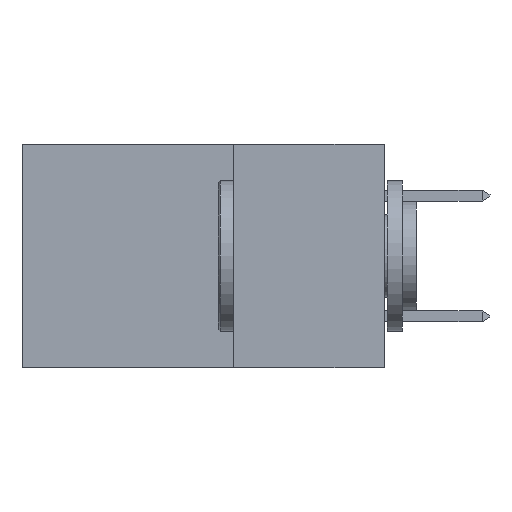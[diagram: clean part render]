
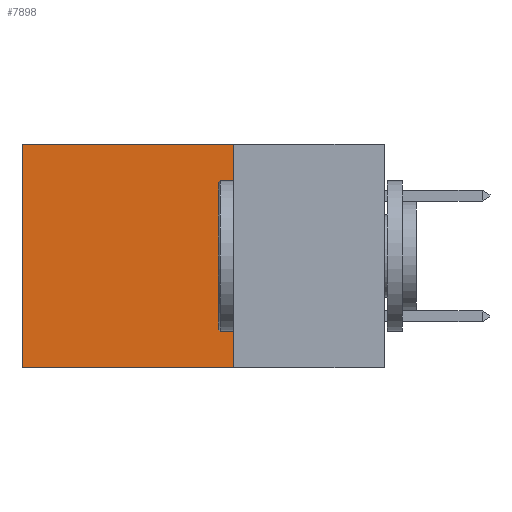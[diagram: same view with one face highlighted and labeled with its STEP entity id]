
A CAD part, left-side view. The second image highlights one B-rep face of the part: STEP entity #7898.
In plain terms, the highlighted planar face has unit normal (-1, 0, 0).
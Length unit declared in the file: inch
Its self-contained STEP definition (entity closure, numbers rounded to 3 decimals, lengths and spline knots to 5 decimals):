
#670 = DIRECTION ( 'NONE',  ( 0., 0., -1. ) ) ;
#1309 = CARTESIAN_POINT ( 'NONE',  ( 0.2875, 0.25, 0. ) ) ;
#4005 = ORIENTED_EDGE ( 'NONE', *, *, #20497, .F. ) ;
#4287 = ORIENTED_EDGE ( 'NONE', *, *, #20809, .T. ) ;
#5944 = ORIENTED_EDGE ( 'NONE', *, *, #7449, .T. ) ;
#6396 = CARTESIAN_POINT ( 'NONE',  ( 0.2875, 0.6, -0.37 ) ) ;
#6902 = LINE ( 'NONE', #20872, #11221 ) ;
#7449 = EDGE_CURVE ( 'NONE', #13087, #17642, #6902, .T. ) ;
#7898 = ADVANCED_FACE ( 'NONE', ( #20900 ), #11120, .F. ) ;
#8577 = VECTOR ( 'NONE', #10182, 39.37008 ) ;
#9138 = ORIENTED_EDGE ( 'NONE', *, *, #9745, .F. ) ;
#9745 = EDGE_CURVE ( 'NONE', #14957, #22148, #23142, .T. ) ;
#9895 = AXIS2_PLACEMENT_3D ( 'NONE', #20223, #23888, #12986 ) ;
#10182 = DIRECTION ( 'NONE',  ( 0., 1., 0. ) ) ;
#11120 = PLANE ( 'NONE',  #9895 ) ;
#11221 = VECTOR ( 'NONE', #13582, 39.37008 ) ;
#11975 = VECTOR ( 'NONE', #16482, 39.37008 ) ;
#12986 = DIRECTION ( 'NONE',  ( 0., 0., -1. ) ) ;
#13087 = VERTEX_POINT ( 'NONE', #1309 ) ;
#13582 = DIRECTION ( 'NONE',  ( 0., 1., 0. ) ) ;
#13696 = CARTESIAN_POINT ( 'NONE',  ( 0.2875, 0.6, 0. ) ) ;
#14343 = CARTESIAN_POINT ( 'NONE',  ( 0.2875, 0.25, -0.37 ) ) ;
#14957 = VERTEX_POINT ( 'NONE', #14343 ) ;
#16482 = DIRECTION ( 'NONE',  ( 0., 0., -1. ) ) ;
#17642 = VERTEX_POINT ( 'NONE', #22409 ) ;
#18065 = EDGE_LOOP ( 'NONE', ( #4287, #9138, #4005, #5944 ) ) ;
#19125 = LINE ( 'NONE', #13696, #23383 ) ;
#19304 = CARTESIAN_POINT ( 'NONE',  ( 0.2875, 0.25, -0.37 ) ) ;
#20068 = CARTESIAN_POINT ( 'NONE',  ( 0.2875, 0.25, 0. ) ) ;
#20223 = CARTESIAN_POINT ( 'NONE',  ( 0.2875, 0.25, 0. ) ) ;
#20497 = EDGE_CURVE ( 'NONE', #13087, #14957, #22264, .T. ) ;
#20809 = EDGE_CURVE ( 'NONE', #17642, #22148, #19125, .T. ) ;
#20872 = CARTESIAN_POINT ( 'NONE',  ( 0.2875, 0.25, 0. ) ) ;
#20900 = FACE_OUTER_BOUND ( 'NONE', #18065, .T. ) ;
#22148 = VERTEX_POINT ( 'NONE', #6396 ) ;
#22264 = LINE ( 'NONE', #20068, #11975 ) ;
#22409 = CARTESIAN_POINT ( 'NONE',  ( 0.2875, 0.6, 0. ) ) ;
#23142 = LINE ( 'NONE', #19304, #8577 ) ;
#23383 = VECTOR ( 'NONE', #670, 39.37008 ) ;
#23888 = DIRECTION ( 'NONE',  ( 1., 0., 0. ) ) ;
